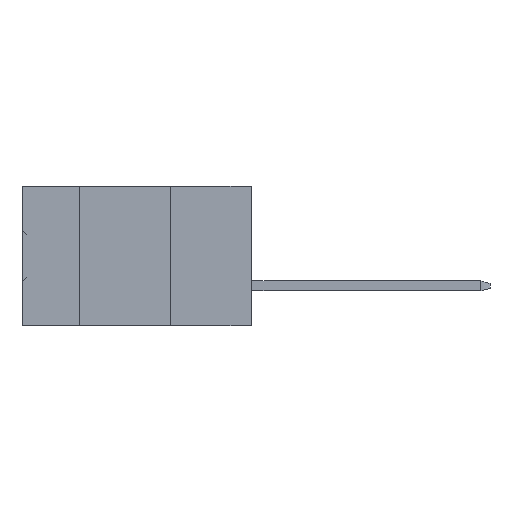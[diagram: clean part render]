
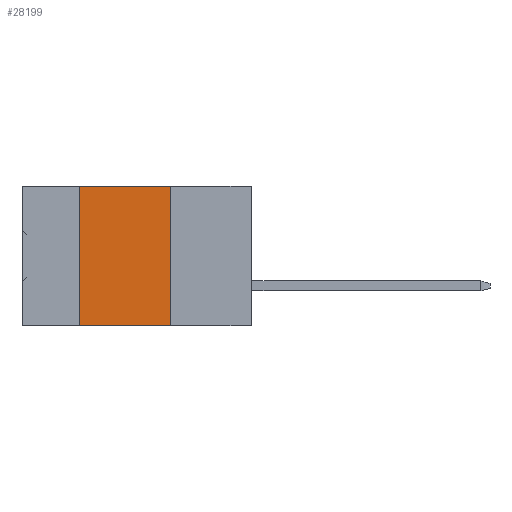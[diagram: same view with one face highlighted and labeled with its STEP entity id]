
A CAD part, left-side view. The second image highlights one B-rep face of the part: STEP entity #28199.
In plain terms, the highlighted planar face has unit normal (-1, 0, 0).
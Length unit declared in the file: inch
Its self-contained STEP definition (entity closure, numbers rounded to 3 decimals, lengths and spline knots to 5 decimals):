
#667 = CARTESIAN_POINT ( 'NONE',  ( 0., 0.254, -0.437 ) ) ;
#1290 = AXIS2_PLACEMENT_3D ( 'NONE', #12581, #10265, #28454 ) ;
#1443 = EDGE_CURVE ( 'NONE', #17272, #29532, #15077, .T. ) ;
#3394 = LINE ( 'NONE', #20156, #28690 ) ;
#3449 = LINE ( 'NONE', #667, #9766 ) ;
#5700 = DIRECTION ( 'NONE',  ( 0., 0., 1. ) ) ;
#7344 = DIRECTION ( 'NONE',  ( 0., -1., 0. ) ) ;
#7806 = PLANE ( 'NONE',  #1290 ) ;
#9634 = LINE ( 'NONE', #19032, #18033 ) ;
#9766 = VECTOR ( 'NONE', #14999, 39.37008 ) ;
#10265 = DIRECTION ( 'NONE',  ( 1., 0., 0. ) ) ;
#10322 = EDGE_CURVE ( 'NONE', #12971, #29532, #3449, .T. ) ;
#10619 = CARTESIAN_POINT ( 'NONE',  ( 0., 0.254, 0. ) ) ;
#12426 = ORIENTED_EDGE ( 'NONE', *, *, #1443, .T. ) ;
#12502 = VERTEX_POINT ( 'NONE', #15756 ) ;
#12581 = CARTESIAN_POINT ( 'NONE',  ( 0., 0.72, 0. ) ) ;
#12971 = VERTEX_POINT ( 'NONE', #10619 ) ;
#13956 = CARTESIAN_POINT ( 'NONE',  ( 0., 0.54, -0.437 ) ) ;
#14999 = DIRECTION ( 'NONE',  ( 0., 0., -1. ) ) ;
#15077 = LINE ( 'NONE', #29400, #16316 ) ;
#15226 = CARTESIAN_POINT ( 'NONE',  ( 0., 0.254, -0.437 ) ) ;
#15756 = CARTESIAN_POINT ( 'NONE',  ( 0., 0.54, 0. ) ) ;
#16316 = VECTOR ( 'NONE', #22755, 39.37008 ) ;
#17210 = FACE_OUTER_BOUND ( 'NONE', #20465, .T. ) ;
#17272 = VERTEX_POINT ( 'NONE', #13956 ) ;
#17459 = EDGE_CURVE ( 'NONE', #17272, #12502, #3394, .T. ) ;
#18033 = VECTOR ( 'NONE', #7344, 39.37008 ) ;
#18699 = ORIENTED_EDGE ( 'NONE', *, *, #17459, .F. ) ;
#19032 = CARTESIAN_POINT ( 'NONE',  ( 0., 0.72, 0. ) ) ;
#20156 = CARTESIAN_POINT ( 'NONE',  ( 0., 0.54, -0.437 ) ) ;
#20465 = EDGE_LOOP ( 'NONE', ( #27967, #27069, #18699, #12426 ) ) ;
#22173 = EDGE_CURVE ( 'NONE', #12502, #12971, #9634, .T. ) ;
#22755 = DIRECTION ( 'NONE',  ( 0., -1., 0. ) ) ;
#27069 = ORIENTED_EDGE ( 'NONE', *, *, #22173, .F. ) ;
#27967 = ORIENTED_EDGE ( 'NONE', *, *, #10322, .F. ) ;
#28199 = ADVANCED_FACE ( 'NONE', ( #17210 ), #7806, .F. ) ;
#28454 = DIRECTION ( 'NONE',  ( 0., 0., -1. ) ) ;
#28690 = VECTOR ( 'NONE', #5700, 39.37008 ) ;
#29400 = CARTESIAN_POINT ( 'NONE',  ( 0., 0.72, -0.437 ) ) ;
#29532 = VERTEX_POINT ( 'NONE', #15226 ) ;
